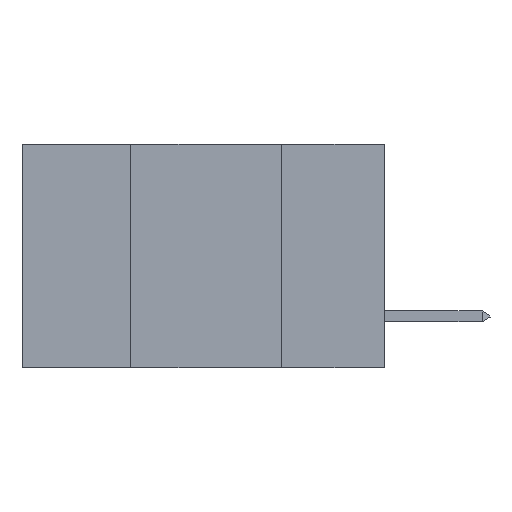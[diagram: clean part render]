
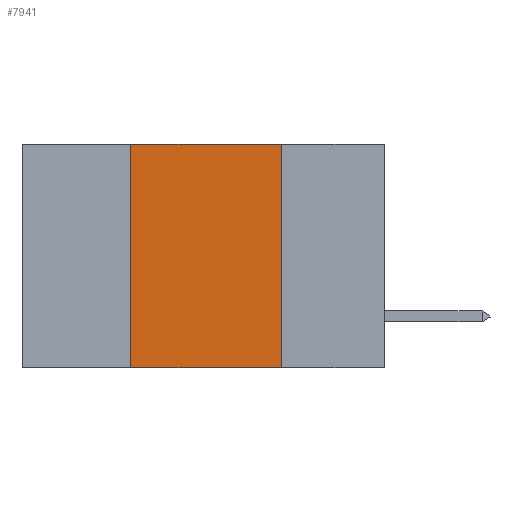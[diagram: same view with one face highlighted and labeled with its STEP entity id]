
A CAD part, left-side view. The second image highlights one B-rep face of the part: STEP entity #7941.
In plain terms, the highlighted planar face has unit normal (-1, 0, 0).
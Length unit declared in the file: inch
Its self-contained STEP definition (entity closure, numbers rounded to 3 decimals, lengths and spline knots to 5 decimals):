
#1007 = VECTOR ( 'NONE', #1572, 39.37008 ) ;
#1055 = EDGE_CURVE ( 'NONE', #12116, #12775, #8220, .T. ) ;
#1274 = CARTESIAN_POINT ( 'NONE',  ( 0., 0.17, 0. ) ) ;
#1554 = DIRECTION ( 'NONE',  ( 0., -1., 0. ) ) ;
#1572 = DIRECTION ( 'NONE',  ( 0., -1., 0. ) ) ;
#2230 = EDGE_CURVE ( 'NONE', #12775, #6043, #10565, .T. ) ;
#2458 = EDGE_LOOP ( 'NONE', ( #2945, #11098, #5714, #6486 ) ) ;
#2597 = EDGE_CURVE ( 'NONE', #12996, #6043, #12278, .T. ) ;
#2676 = LINE ( 'NONE', #6164, #3379 ) ;
#2945 = ORIENTED_EDGE ( 'NONE', *, *, #2230, .F. ) ;
#2952 = DIRECTION ( 'NONE',  ( 0., 0., -1. ) ) ;
#2997 = DIRECTION ( 'NONE',  ( 1., 0., 0. ) ) ;
#3379 = VECTOR ( 'NONE', #13710, 39.37008 ) ;
#3561 = EDGE_CURVE ( 'NONE', #12996, #12116, #2676, .T. ) ;
#3595 = FACE_OUTER_BOUND ( 'NONE', #2458, .T. ) ;
#4766 = CARTESIAN_POINT ( 'NONE',  ( 0., 0.17, 0. ) ) ;
#4873 = CARTESIAN_POINT ( 'NONE',  ( 0., 0.6, 0. ) ) ;
#5639 = AXIS2_PLACEMENT_3D ( 'NONE', #13667, #2997, #2952 ) ;
#5714 = ORIENTED_EDGE ( 'NONE', *, *, #3561, .F. ) ;
#6043 = VERTEX_POINT ( 'NONE', #13831 ) ;
#6083 = CARTESIAN_POINT ( 'NONE',  ( 0., 0.42, 0. ) ) ;
#6164 = CARTESIAN_POINT ( 'NONE',  ( 0., 0.42, 0. ) ) ;
#6486 = ORIENTED_EDGE ( 'NONE', *, *, #2597, .T. ) ;
#6848 = VECTOR ( 'NONE', #13399, 39.37008 ) ;
#7941 = ADVANCED_FACE ( 'NONE', ( #3595 ), #10204, .F. ) ;
#8220 = LINE ( 'NONE', #4873, #1007 ) ;
#10204 = PLANE ( 'NONE',  #5639 ) ;
#10565 = LINE ( 'NONE', #4766, #6848 ) ;
#11098 = ORIENTED_EDGE ( 'NONE', *, *, #1055, .F. ) ;
#12116 = VERTEX_POINT ( 'NONE', #6083 ) ;
#12278 = LINE ( 'NONE', #13691, #13591 ) ;
#12775 = VERTEX_POINT ( 'NONE', #1274 ) ;
#12996 = VERTEX_POINT ( 'NONE', #13531 ) ;
#13399 = DIRECTION ( 'NONE',  ( 0., 0., -1. ) ) ;
#13531 = CARTESIAN_POINT ( 'NONE',  ( 0., 0.42, -0.37 ) ) ;
#13591 = VECTOR ( 'NONE', #1554, 39.37008 ) ;
#13667 = CARTESIAN_POINT ( 'NONE',  ( 0., 0.6, 0. ) ) ;
#13691 = CARTESIAN_POINT ( 'NONE',  ( 0., 0.6, -0.37 ) ) ;
#13710 = DIRECTION ( 'NONE',  ( 0., 0., 1. ) ) ;
#13831 = CARTESIAN_POINT ( 'NONE',  ( 0., 0.17, -0.37 ) ) ;
